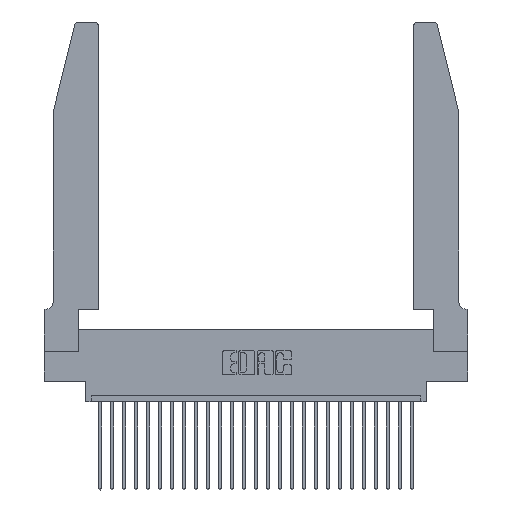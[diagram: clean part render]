
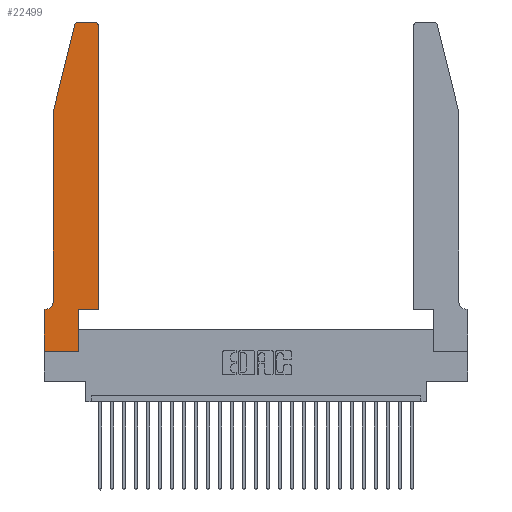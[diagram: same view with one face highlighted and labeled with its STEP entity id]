
A CAD part, top view. The second image highlights one B-rep face of the part: STEP entity #22499.
In plain terms, the highlighted planar face has unit normal (0, 0, 1).
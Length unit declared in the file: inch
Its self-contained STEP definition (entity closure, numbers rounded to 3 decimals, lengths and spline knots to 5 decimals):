
#821 = EDGE_CURVE ( 'NONE', #18136, #11907, #24535, .T. ) ;
#1153 = CARTESIAN_POINT ( 'NONE',  ( 0., 0., 0.37 ) ) ;
#1291 = ORIENTED_EDGE ( 'NONE', *, *, #16260, .T. ) ;
#1300 = VECTOR ( 'NONE', #5055, 39.37008 ) ;
#1372 = LINE ( 'NONE', #21781, #2025 ) ;
#1613 = CARTESIAN_POINT ( 'NONE',  ( 0.284, 2.72, 0.37 ) ) ;
#2025 = VECTOR ( 'NONE', #3023, 39.37008 ) ;
#2130 = EDGE_CURVE ( 'NONE', #13080, #5184, #26516, .T. ) ;
#2181 = LINE ( 'NONE', #25297, #25822 ) ;
#2193 = DIRECTION ( 'NONE',  ( 0., 0., -1. ) ) ;
#2212 = ORIENTED_EDGE ( 'NONE', *, *, #821, .T. ) ;
#2693 = EDGE_CURVE ( 'NONE', #11907, #13080, #10709, .T. ) ;
#3023 = DIRECTION ( 'NONE',  ( 1., 0., 0. ) ) ;
#3546 = VECTOR ( 'NONE', #8252, 39.37008 ) ;
#3724 = DIRECTION ( 'NONE',  ( 1., 0., 0. ) ) ;
#3966 = CARTESIAN_POINT ( 'NONE',  ( 0.2865, 0.35, 0.37 ) ) ;
#4072 = VECTOR ( 'NONE', #8422, 39.37008 ) ;
#4183 = CARTESIAN_POINT ( 'NONE',  ( 0.284, 2.75, 0.37 ) ) ;
#4249 = CARTESIAN_POINT ( 'NONE',  ( 0.0055, 0.42, 0.37 ) ) ;
#4371 = CARTESIAN_POINT ( 'NONE',  ( 0.0755, 0.42, 0.37 ) ) ;
#4683 = VERTEX_POINT ( 'NONE', #8321 ) ;
#4748 = AXIS2_PLACEMENT_3D ( 'NONE', #4249, #2193, #6339 ) ;
#5055 = DIRECTION ( 'NONE',  ( 0., -1., 0. ) ) ;
#5106 = VERTEX_POINT ( 'NONE', #1153 ) ;
#5143 = VERTEX_POINT ( 'NONE', #20033 ) ;
#5184 = VERTEX_POINT ( 'NONE', #24255 ) ;
#5283 = ORIENTED_EDGE ( 'NONE', *, *, #23728, .T. ) ;
#6237 = CARTESIAN_POINT ( 'NONE',  ( 0.4205, 2.72, 0.37 ) ) ;
#6339 = DIRECTION ( 'NONE',  ( -1., 0., 0. ) ) ;
#6445 = AXIS2_PLACEMENT_3D ( 'NONE', #1613, #12356, #22607 ) ;
#6579 = CARTESIAN_POINT ( 'NONE',  ( 0.4205, 2.75, 0.37 ) ) ;
#6890 = VECTOR ( 'NONE', #23281, 39.37008 ) ;
#7242 = ORIENTED_EDGE ( 'NONE', *, *, #8694, .T. ) ;
#7708 = CARTESIAN_POINT ( 'NONE',  ( 0.4505, 0.35, 0.37 ) ) ;
#8252 = DIRECTION ( 'NONE',  ( -0.239, -0.971, 0. ) ) ;
#8321 = CARTESIAN_POINT ( 'NONE',  ( 0.2865, 0.35, 0.37 ) ) ;
#8422 = DIRECTION ( 'NONE',  ( -1., 0., 0. ) ) ;
#8694 = EDGE_CURVE ( 'NONE', #24748, #23157, #11617, .T. ) ;
#9422 = ORIENTED_EDGE ( 'NONE', *, *, #2693, .T. ) ;
#9700 = EDGE_CURVE ( 'NONE', #5106, #14329, #1372, .T. ) ;
#9933 = DIRECTION ( 'NONE',  ( 0., 1., 0. ) ) ;
#10500 = LINE ( 'NONE', #17595, #1300 ) ;
#10651 = DIRECTION ( 'NONE',  ( 0., 0., 1. ) ) ;
#10709 = CIRCLE ( 'NONE', #6445, 0.03 ) ;
#10755 = VECTOR ( 'NONE', #13379, 39.37008 ) ;
#11283 = EDGE_LOOP ( 'NONE', ( #2212, #9422, #27007, #1291, #26969, #7242, #20481, #24068, #17402, #22328, #12503, #5283 ) ) ;
#11617 = LINE ( 'NONE', #16768, #4072 ) ;
#11889 = VERTEX_POINT ( 'NONE', #4371 ) ;
#11907 = VERTEX_POINT ( 'NONE', #4183 ) ;
#12143 = CARTESIAN_POINT ( 'NONE',  ( 0., 0.35, 0.37 ) ) ;
#12206 = VERTEX_POINT ( 'NONE', #25330 ) ;
#12356 = DIRECTION ( 'NONE',  ( 0., 0., 1. ) ) ;
#12419 = CIRCLE ( 'NONE', #13708, 0.03 ) ;
#12427 = EDGE_CURVE ( 'NONE', #4683, #12206, #2181, .T. ) ;
#12503 = ORIENTED_EDGE ( 'NONE', *, *, #16014, .T. ) ;
#12742 = DIRECTION ( 'NONE',  ( 1., 0., 0. ) ) ;
#13080 = VERTEX_POINT ( 'NONE', #14301 ) ;
#13149 = VECTOR ( 'NONE', #9933, 39.37008 ) ;
#13379 = DIRECTION ( 'NONE',  ( -1., 0., 0. ) ) ;
#13708 = AXIS2_PLACEMENT_3D ( 'NONE', #6237, #10651, #25016 ) ;
#13964 = CARTESIAN_POINT ( 'NONE',  ( 0.2865, 0., 0.37 ) ) ;
#14301 = CARTESIAN_POINT ( 'NONE',  ( 0.25487, 2.72718, 0.37 ) ) ;
#14329 = VERTEX_POINT ( 'NONE', #13964 ) ;
#14587 = EDGE_CURVE ( 'NONE', #14329, #4683, #18053, .T. ) ;
#14715 = CARTESIAN_POINT ( 'NONE',  ( 0., 0.35, 0.37 ) ) ;
#15126 = LINE ( 'NONE', #7708, #13149 ) ;
#16014 = EDGE_CURVE ( 'NONE', #12206, #5143, #15126, .T. ) ;
#16260 = EDGE_CURVE ( 'NONE', #5184, #11889, #10500, .T. ) ;
#16768 = CARTESIAN_POINT ( 'NONE',  ( 0.0755, 0.35, 0.37 ) ) ;
#16977 = LINE ( 'NONE', #18504, #22878 ) ;
#17402 = ORIENTED_EDGE ( 'NONE', *, *, #14587, .T. ) ;
#17595 = CARTESIAN_POINT ( 'NONE',  ( 0.0755, 2., 0.37 ) ) ;
#18053 = LINE ( 'NONE', #3966, #6890 ) ;
#18136 = VERTEX_POINT ( 'NONE', #6579 ) ;
#18504 = CARTESIAN_POINT ( 'NONE',  ( 0., 0., 0.37 ) ) ;
#18618 = DIRECTION ( 'NONE',  ( 0., 0., 1. ) ) ;
#20033 = CARTESIAN_POINT ( 'NONE',  ( 0.4505, 2.72, 0.37 ) ) ;
#20085 = CARTESIAN_POINT ( 'NONE',  ( 0.0055, 0.35, 0.37 ) ) ;
#20481 = ORIENTED_EDGE ( 'NONE', *, *, #26288, .T. ) ;
#20604 = DIRECTION ( 'NONE',  ( 0., -1., 0. ) ) ;
#20763 = CARTESIAN_POINT ( 'NONE',  ( 0.0755, 2., 0.37 ) ) ;
#21249 = CIRCLE ( 'NONE', #4748, 0.07 ) ;
#21781 = CARTESIAN_POINT ( 'NONE',  ( 0., 0., 0.37 ) ) ;
#21884 = CARTESIAN_POINT ( 'NONE',  ( 0.2605, 2.75, 0.37 ) ) ;
#22328 = ORIENTED_EDGE ( 'NONE', *, *, #12427, .T. ) ;
#22499 = ADVANCED_FACE ( 'NONE', ( #25620 ), #24605, .T. ) ;
#22607 = DIRECTION ( 'NONE',  ( 1., 0., 0. ) ) ;
#22878 = VECTOR ( 'NONE', #20604, 39.37008 ) ;
#23157 = VERTEX_POINT ( 'NONE', #14715 ) ;
#23281 = DIRECTION ( 'NONE',  ( 0., 1., 0. ) ) ;
#23681 = AXIS2_PLACEMENT_3D ( 'NONE', #12143, #18618, #3724 ) ;
#23728 = EDGE_CURVE ( 'NONE', #5143, #18136, #12419, .T. ) ;
#23800 = EDGE_CURVE ( 'NONE', #11889, #24748, #21249, .T. ) ;
#24068 = ORIENTED_EDGE ( 'NONE', *, *, #9700, .T. ) ;
#24255 = CARTESIAN_POINT ( 'NONE',  ( 0.0755, 2., 0.37 ) ) ;
#24535 = LINE ( 'NONE', #21884, #10755 ) ;
#24605 = PLANE ( 'NONE',  #23681 ) ;
#24748 = VERTEX_POINT ( 'NONE', #20085 ) ;
#25016 = DIRECTION ( 'NONE',  ( 1., 0., 0. ) ) ;
#25297 = CARTESIAN_POINT ( 'NONE',  ( 0.4505, 0.35, 0.37 ) ) ;
#25330 = CARTESIAN_POINT ( 'NONE',  ( 0.4505, 0.35, 0.37 ) ) ;
#25620 = FACE_OUTER_BOUND ( 'NONE', #11283, .T. ) ;
#25822 = VECTOR ( 'NONE', #12742, 39.37008 ) ;
#26288 = EDGE_CURVE ( 'NONE', #23157, #5106, #16977, .T. ) ;
#26516 = LINE ( 'NONE', #20763, #3546 ) ;
#26969 = ORIENTED_EDGE ( 'NONE', *, *, #23800, .T. ) ;
#27007 = ORIENTED_EDGE ( 'NONE', *, *, #2130, .T. ) ;
